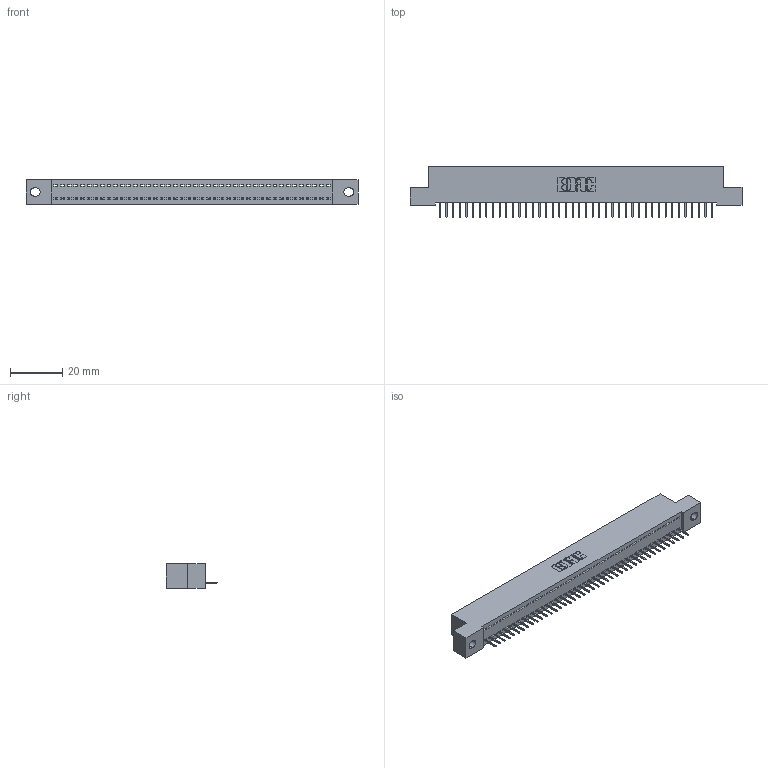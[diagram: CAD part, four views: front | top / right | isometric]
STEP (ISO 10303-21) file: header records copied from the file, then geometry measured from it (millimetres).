
FILE_DESCRIPTION (( 'STEP AP203' ), '1' );
FILE_NAME ('392-042-524-102.STEP', '2019-10-07T20:58:28', ( '' ), ( '' ), 'SwSTEP 2.0', 'SolidWorks 2016', '' );
FILE_SCHEMA (( 'CONFIG_CONTROL_DESIGN' ));
Length unit declared in the file: inch
Products named in the file (3): 342 Part_.128 Slot; 392-042-524-102; 345-292-001_345-293-124
Assembly tree (43 placements, depth 2):
  392-042-524-102
    342 Part_.128 Slot
    345-292-001_345-293-124  x42
Bounding box: 127 x 19.69 x 9.4 mm (x, y, z)
Volume: 10917.3 mm3; surface area: 15275.9 mm2
Topology: 43 solids, 43 shells, 2718 faces, 7871 edges, 5078 vertices
Faces by surface type: plane 2086, cylinder 632
Entity records: 25753 total; most frequent: CARTESIAN_POINT 4448, ORIENTED_EDGE 4426, DIRECTION 3753, EDGE_CURVE 2213, VECTOR 2089, LINE 2089, VERTEX_POINT 1470, AXIS2_PLACEMENT_3D 832
